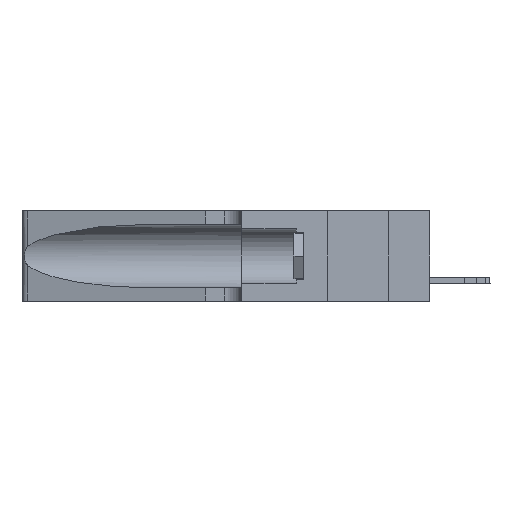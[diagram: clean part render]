
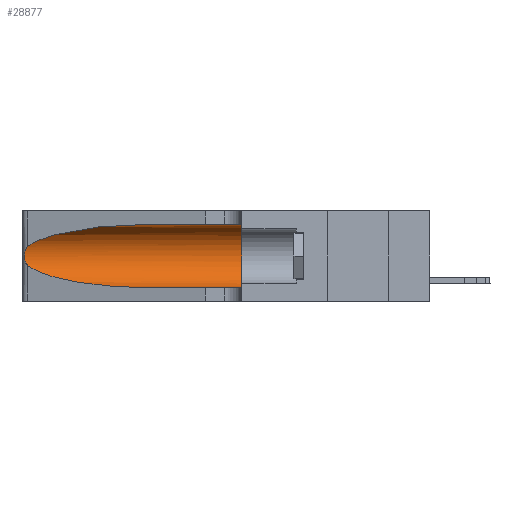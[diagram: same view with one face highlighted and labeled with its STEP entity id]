
A CAD part, left-side view. The second image highlights one B-rep face of the part: STEP entity #28877.
In plain terms, the highlighted cylindrical face has radius 3.308 mm (diameter 6.617 mm), a partial arc.
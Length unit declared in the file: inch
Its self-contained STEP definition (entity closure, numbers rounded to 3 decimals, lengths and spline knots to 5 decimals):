
#173 = DIRECTION ( 'NONE',  ( 0., -1., 0. ) ) ;
#4078 = CIRCLE ( 'NONE', #28913, 0.13025 ) ;
#4647 = B_SPLINE_CURVE_WITH_KNOTS ( 'NONE', 3,
 ( #15592, #8467, #18465, #15835, #25285, #11237, #25397, #19844, #22809, #11133, #28978, #6222, #17768, #9048 ),
 .UNSPECIFIED., .F., .F.,
 ( 4, 2, 2, 2, 2, 2, 4 ),
 ( 0., 0.00027, 0.00053, 0.00107, 0.0016, 0.00187, 0.00214 ),
 .UNSPECIFIED. ) ;
#5073 = LINE ( 'NONE', #34667, #13767 ) ;
#5579 = VERTEX_POINT ( 'NONE', #26683 ) ;
#6222 = CARTESIAN_POINT ( 'NONE',  ( 0.25639, 1.23186, 0.15144 ) ) ;
#6354 = DIRECTION ( 'NONE',  ( 0., 0., -1. ) ) ;
#6818 = VERTEX_POINT ( 'NONE', #21247 ) ;
#7440 = CARTESIAN_POINT ( 'NONE',  ( 0.18966, 0.96281, 0.05475 ) ) ;
#7906 = EDGE_LOOP ( 'NONE', ( #26521, #29876, #19604, #13583, #23353, #9809 ) ) ;
#8083 = CARTESIAN_POINT ( 'NONE',  ( 0.1305, 0.35, 0.05475 ) ) ;
#8467 = CARTESIAN_POINT ( 'NONE',  ( 0.25555, 1.22994, 0.2215 ) ) ;
#8914 = VERTEX_POINT ( 'NONE', #18643 ) ;
#9048 = CARTESIAN_POINT ( 'NONE',  ( 0.25487, 1.22718, 0.14631 ) ) ;
#9164 = DIRECTION ( 'NONE',  ( 0., -1., 0. ) ) ;
#9801 = EDGE_CURVE ( 'NONE', #30155, #24881, #5073, .T. ) ;
#9809 = ORIENTED_EDGE ( 'NONE', *, *, #28367, .F. ) ;
#11133 = CARTESIAN_POINT ( 'NONE',  ( 0.25856, 1.23593, 0.16098 ) ) ;
#11221 = CARTESIAN_POINT ( 'NONE',  ( 0.1305, 0.35, 0.185 ) ) ;
#11237 = CARTESIAN_POINT ( 'NONE',  ( 0.26018, 1.23835, 0.19895 ) ) ;
#11550 = EDGE_CURVE ( 'NONE', #5579, #8914, #24189, .T. ) ;
#12834 = CARTESIAN_POINT ( 'NONE',  ( 0.1305, 0.72297, 0.05475 ) ) ;
#12966 = CARTESIAN_POINT ( 'NONE',  ( 0.2373, 1.15595, 0.08982 ) ) ;
#13583 = ORIENTED_EDGE ( 'NONE', *, *, #9801, .T. ) ;
#13767 = VECTOR ( 'NONE', #9164, 39.37008 ) ;
#15191 = AXIS2_PLACEMENT_3D ( 'NONE', #33147, #173, #6354 ) ;
#15592 = CARTESIAN_POINT ( 'NONE',  ( 0.25487, 1.22718, 0.22369 ) ) ;
#15835 = CARTESIAN_POINT ( 'NONE',  ( 0.25787, 1.23484, 0.2124 ) ) ;
#17661 = EDGE_CURVE ( 'NONE', #8914, #25158, #4647, .T. ) ;
#17768 = CARTESIAN_POINT ( 'NONE',  ( 0.25555, 1.22993, 0.14849 ) ) ;
#18465 = CARTESIAN_POINT ( 'NONE',  ( 0.25639, 1.23184, 0.21858 ) ) ;
#18643 = CARTESIAN_POINT ( 'NONE',  ( 0.25487, 1.22718, 0.22369 ) ) ;
#19604 = ORIENTED_EDGE ( 'NONE', *, *, #20673, .T. ) ;
#19844 = CARTESIAN_POINT ( 'NONE',  ( 0.26075, 1.23896, 0.178 ) ) ;
#19947 = CARTESIAN_POINT ( 'NONE',  ( 0.1305, 1.61858, 0.31525 ) ) ;
#20367 =( BOUNDED_CURVE ( )  B_SPLINE_CURVE ( 3, ( #20980, #12966, #7440, #12834 ),
 .UNSPECIFIED., .F., .F. ) 
 B_SPLINE_CURVE_WITH_KNOTS ( ( 4, 4 ),
 ( 3.44316, 4.71239 ),
 .UNSPECIFIED. ) 
 CURVE ( )  GEOMETRIC_REPRESENTATION_ITEM ( )  RATIONAL_B_SPLINE_CURVE ( ( 1., 0.87, 0.87, 1. ) ) 
 REPRESENTATION_ITEM ( '' )  );
#20673 = EDGE_CURVE ( 'NONE', #25158, #30155, #20367, .T. ) ;
#20980 = CARTESIAN_POINT ( 'NONE',  ( 0.25487, 1.22718, 0.14631 ) ) ;
#21247 = CARTESIAN_POINT ( 'NONE',  ( 0.1305, 0.35, 0.31525 ) ) ;
#22560 = DIRECTION ( 'NONE',  ( 0., 1., 0. ) ) ;
#22741 = VECTOR ( 'NONE', #25853, 39.37008 ) ;
#22809 = CARTESIAN_POINT ( 'NONE',  ( 0.26017, 1.23833, 0.17102 ) ) ;
#23353 = ORIENTED_EDGE ( 'NONE', *, *, #28330, .F. ) ;
#24189 =( BOUNDED_CURVE ( )  B_SPLINE_CURVE ( 3, ( #34280, #25991, #34402, #28491 ),
 .UNSPECIFIED., .F., .F. ) 
 B_SPLINE_CURVE_WITH_KNOTS ( ( 4, 4 ),
 ( 1.5708, 2.84003 ),
 .UNSPECIFIED. ) 
 CURVE ( )  GEOMETRIC_REPRESENTATION_ITEM ( )  RATIONAL_B_SPLINE_CURVE ( ( 1., 0.87, 0.87, 1. ) ) 
 REPRESENTATION_ITEM ( '' )  );
#24575 = LINE ( 'NONE', #19947, #22741 ) ;
#24868 = FACE_OUTER_BOUND ( 'NONE', #7906, .T. ) ;
#24881 = VERTEX_POINT ( 'NONE', #8083 ) ;
#25158 = VERTEX_POINT ( 'NONE', #32400 ) ;
#25285 = CARTESIAN_POINT ( 'NONE',  ( 0.25854, 1.2359, 0.20912 ) ) ;
#25397 = CARTESIAN_POINT ( 'NONE',  ( 0.26075, 1.23896, 0.19203 ) ) ;
#25853 = DIRECTION ( 'NONE',  ( 0., -1., 0. ) ) ;
#25991 = CARTESIAN_POINT ( 'NONE',  ( 0.18966, 0.96281, 0.31525 ) ) ;
#26168 = CYLINDRICAL_SURFACE ( 'NONE', #15191, 0.13025 ) ;
#26521 = ORIENTED_EDGE ( 'NONE', *, *, #11550, .T. ) ;
#26683 = CARTESIAN_POINT ( 'NONE',  ( 0.1305, 0.72297, 0.31525 ) ) ;
#28330 = EDGE_CURVE ( 'NONE', #6818, #24881, #4078, .T. ) ;
#28367 = EDGE_CURVE ( 'NONE', #5579, #6818, #24575, .T. ) ;
#28491 = CARTESIAN_POINT ( 'NONE',  ( 0.25487, 1.22718, 0.22369 ) ) ;
#28877 = ADVANCED_FACE ( 'NONE', ( #24868 ), #26168, .F. ) ;
#28913 = AXIS2_PLACEMENT_3D ( 'NONE', #11221, #22560, #36169 ) ;
#28978 = CARTESIAN_POINT ( 'NONE',  ( 0.25789, 1.23486, 0.15765 ) ) ;
#29671 = CARTESIAN_POINT ( 'NONE',  ( 0.1305, 0.72297, 0.05475 ) ) ;
#29876 = ORIENTED_EDGE ( 'NONE', *, *, #17661, .T. ) ;
#30155 = VERTEX_POINT ( 'NONE', #29671 ) ;
#32400 = CARTESIAN_POINT ( 'NONE',  ( 0.25487, 1.22718, 0.14631 ) ) ;
#33147 = CARTESIAN_POINT ( 'NONE',  ( 0.1305, 1.61858, 0.185 ) ) ;
#34280 = CARTESIAN_POINT ( 'NONE',  ( 0.1305, 0.72297, 0.31525 ) ) ;
#34402 = CARTESIAN_POINT ( 'NONE',  ( 0.2373, 1.15595, 0.28018 ) ) ;
#34667 = CARTESIAN_POINT ( 'NONE',  ( 0.1305, 1.61858, 0.05475 ) ) ;
#36169 = DIRECTION ( 'NONE',  ( 0., 0., 1. ) ) ;
